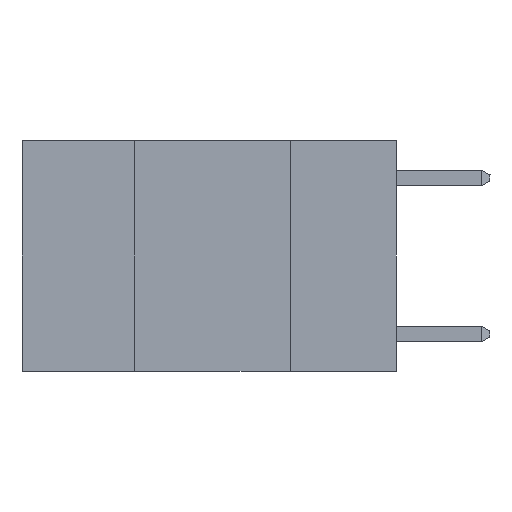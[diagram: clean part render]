
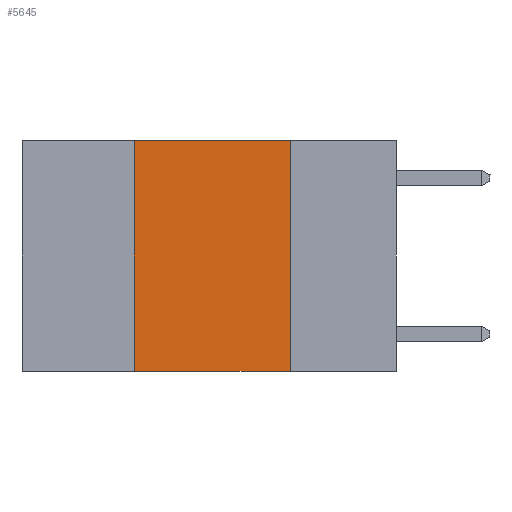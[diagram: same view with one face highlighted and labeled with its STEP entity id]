
A CAD part, left-side view. The second image highlights one B-rep face of the part: STEP entity #5645.
In plain terms, the highlighted planar face has unit normal (-1, 0, 0).
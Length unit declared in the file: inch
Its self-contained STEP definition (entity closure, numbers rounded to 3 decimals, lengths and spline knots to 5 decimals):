
#61 = ORIENTED_EDGE ( 'NONE', *, *, #1050, .F. ) ;
#165 = EDGE_CURVE ( 'NONE', #7475, #974, #1267, .T. ) ;
#195 = FACE_OUTER_BOUND ( 'NONE', #1669, .T. ) ;
#301 = EDGE_CURVE ( 'NONE', #418, #7906, #1216, .T. ) ;
#418 = VERTEX_POINT ( 'NONE', #8094 ) ;
#488 = CARTESIAN_POINT ( 'NONE',  ( 0., 0.6, -0.37 ) ) ;
#756 = ORIENTED_EDGE ( 'NONE', *, *, #165, .F. ) ;
#974 = VERTEX_POINT ( 'NONE', #2978 ) ;
#985 = LINE ( 'NONE', #8195, #3079 ) ;
#1050 = EDGE_CURVE ( 'NONE', #974, #7906, #985, .T. ) ;
#1098 = ORIENTED_EDGE ( 'NONE', *, *, #301, .T. ) ;
#1216 = LINE ( 'NONE', #488, #5711 ) ;
#1267 = LINE ( 'NONE', #1417, #1377 ) ;
#1377 = VECTOR ( 'NONE', #4994, 39.37008 ) ;
#1417 = CARTESIAN_POINT ( 'NONE',  ( 0., 0.6, 0. ) ) ;
#1669 = EDGE_LOOP ( 'NONE', ( #61, #756, #5037, #1098 ) ) ;
#2710 = DIRECTION ( 'NONE',  ( 0., -1., 0. ) ) ;
#2978 = CARTESIAN_POINT ( 'NONE',  ( 0., 0.17, 0. ) ) ;
#3048 = CARTESIAN_POINT ( 'NONE',  ( 0., 0.17, -0.37 ) ) ;
#3079 = VECTOR ( 'NONE', #5330, 39.37008 ) ;
#4952 = LINE ( 'NONE', #6351, #7022 ) ;
#4994 = DIRECTION ( 'NONE',  ( 0., -1., 0. ) ) ;
#5037 = ORIENTED_EDGE ( 'NONE', *, *, #5246, .F. ) ;
#5246 = EDGE_CURVE ( 'NONE', #418, #7475, #4952, .T. ) ;
#5330 = DIRECTION ( 'NONE',  ( 0., 0., -1. ) ) ;
#5645 = ADVANCED_FACE ( 'NONE', ( #195 ), #8386, .F. ) ;
#5711 = VECTOR ( 'NONE', #2710, 39.37008 ) ;
#6092 = AXIS2_PLACEMENT_3D ( 'NONE', #6102, #6928, #9072 ) ;
#6102 = CARTESIAN_POINT ( 'NONE',  ( 0., 0.6, 0. ) ) ;
#6351 = CARTESIAN_POINT ( 'NONE',  ( 0., 0.42, 0. ) ) ;
#6928 = DIRECTION ( 'NONE',  ( 1., 0., 0. ) ) ;
#7022 = VECTOR ( 'NONE', #7894, 39.37008 ) ;
#7475 = VERTEX_POINT ( 'NONE', #7705 ) ;
#7705 = CARTESIAN_POINT ( 'NONE',  ( 0., 0.42, 0. ) ) ;
#7894 = DIRECTION ( 'NONE',  ( 0., 0., 1. ) ) ;
#7906 = VERTEX_POINT ( 'NONE', #3048 ) ;
#8094 = CARTESIAN_POINT ( 'NONE',  ( 0., 0.42, -0.37 ) ) ;
#8195 = CARTESIAN_POINT ( 'NONE',  ( 0., 0.17, 0. ) ) ;
#8386 = PLANE ( 'NONE',  #6092 ) ;
#9072 = DIRECTION ( 'NONE',  ( 0., 0., -1. ) ) ;
